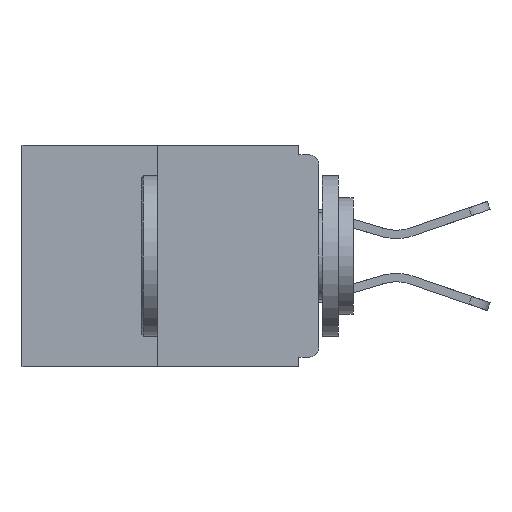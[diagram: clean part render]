
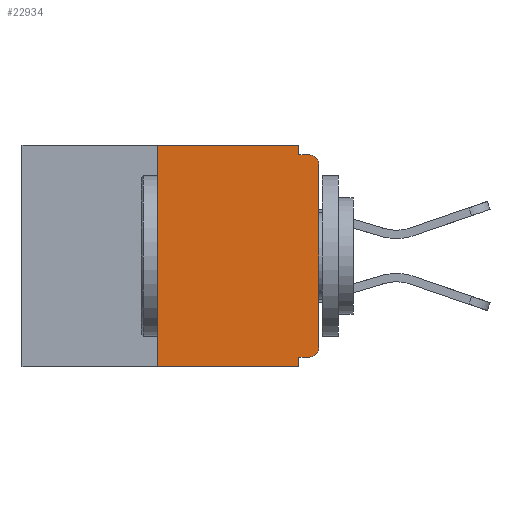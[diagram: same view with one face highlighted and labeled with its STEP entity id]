
A CAD part, left-side view. The second image highlights one B-rep face of the part: STEP entity #22934.
In plain terms, the highlighted planar face has unit normal (-1, 0, 0).
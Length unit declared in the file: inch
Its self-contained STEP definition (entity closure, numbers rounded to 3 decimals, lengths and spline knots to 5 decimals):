
#298 = ORIENTED_EDGE ( 'NONE', *, *, #27920, .F. ) ;
#643 = AXIS2_PLACEMENT_3D ( 'NONE', #21522, #7256, #24028 ) ;
#1594 = EDGE_CURVE ( 'NONE', #24351, #18713, #19865, .T. ) ;
#2471 = DIRECTION ( 'NONE',  ( 0., 0., 1. ) ) ;
#2542 = CARTESIAN_POINT ( 'NONE',  ( 0., 0., -0.015 ) ) ;
#2867 = CARTESIAN_POINT ( 'NONE',  ( 0., 0.46, -0.343 ) ) ;
#2940 = CARTESIAN_POINT ( 'NONE',  ( 0., 0.25, 0. ) ) ;
#3833 = VECTOR ( 'NONE', #12038, 39.37008 ) ;
#4502 = VERTEX_POINT ( 'NONE', #25814 ) ;
#4508 = DIRECTION ( 'NONE',  ( 0., 0., -1. ) ) ;
#5041 = LINE ( 'NONE', #2867, #21056 ) ;
#5176 = CARTESIAN_POINT ( 'NONE',  ( 0., 0., -0.328 ) ) ;
#5350 = LINE ( 'NONE', #2542, #3833 ) ;
#5552 = DIRECTION ( 'NONE',  ( 0., -1., 0. ) ) ;
#6161 = LINE ( 'NONE', #13397, #23680 ) ;
#6518 = EDGE_LOOP ( 'NONE', ( #11911, #21183, #27392, #6928, #298, #19689, #8273, #9486, #28168, #14621 ) ) ;
#6821 = VERTEX_POINT ( 'NONE', #10966 ) ;
#6928 = ORIENTED_EDGE ( 'NONE', *, *, #21513, .F. ) ;
#6950 = DIRECTION ( 'NONE',  ( -1., 0., 0. ) ) ;
#7131 = CARTESIAN_POINT ( 'NONE',  ( 0., 0., 0. ) ) ;
#7256 = DIRECTION ( 'NONE',  ( -1., 0., 0. ) ) ;
#7584 = VECTOR ( 'NONE', #14954, 39.37008 ) ;
#8237 = VERTEX_POINT ( 'NONE', #13868 ) ;
#8273 = ORIENTED_EDGE ( 'NONE', *, *, #19699, .T. ) ;
#8434 = CARTESIAN_POINT ( 'NONE',  ( 0., 0.015, -0.015 ) ) ;
#8556 = CARTESIAN_POINT ( 'NONE',  ( 0., 0.031, 0. ) ) ;
#8578 = CARTESIAN_POINT ( 'NONE',  ( 0., 0.46, 0. ) ) ;
#8872 = VERTEX_POINT ( 'NONE', #19354 ) ;
#9145 = CARTESIAN_POINT ( 'NONE',  ( 0., 0., -0.03 ) ) ;
#9486 = ORIENTED_EDGE ( 'NONE', *, *, #30631, .T. ) ;
#9489 = LINE ( 'NONE', #7131, #19171 ) ;
#10614 = VERTEX_POINT ( 'NONE', #28430 ) ;
#10966 = CARTESIAN_POINT ( 'NONE',  ( 0., 0., -0.313 ) ) ;
#11784 = EDGE_CURVE ( 'NONE', #19048, #8872, #14375, .T. ) ;
#11911 = ORIENTED_EDGE ( 'NONE', *, *, #26491, .F. ) ;
#11927 = CIRCLE ( 'NONE', #643, 0.015 ) ;
#12038 = DIRECTION ( 'NONE',  ( 0., -1., 0. ) ) ;
#12622 = DIRECTION ( 'NONE',  ( 0., 1., 0. ) ) ;
#13140 = CARTESIAN_POINT ( 'NONE',  ( 0., 0.25, 0. ) ) ;
#13221 = AXIS2_PLACEMENT_3D ( 'NONE', #21212, #6950, #23631 ) ;
#13397 = CARTESIAN_POINT ( 'NONE',  ( 0., 0.031, -0.343 ) ) ;
#13868 = CARTESIAN_POINT ( 'NONE',  ( 0., 0.031, -0.343 ) ) ;
#14261 = VERTEX_POINT ( 'NONE', #9145 ) ;
#14375 = LINE ( 'NONE', #15808, #20764 ) ;
#14544 = LINE ( 'NONE', #5176, #19390 ) ;
#14621 = ORIENTED_EDGE ( 'NONE', *, *, #11784, .F. ) ;
#14954 = DIRECTION ( 'NONE',  ( 0., 0., 1. ) ) ;
#15428 = DIRECTION ( 'NONE',  ( 0., 0., -1. ) ) ;
#15533 = DIRECTION ( 'NONE',  ( 1., 0., 0. ) ) ;
#15808 = CARTESIAN_POINT ( 'NONE',  ( 0., 0.031, 0. ) ) ;
#16171 = CARTESIAN_POINT ( 'NONE',  ( 0., 0.46, 0. ) ) ;
#17566 = CARTESIAN_POINT ( 'NONE',  ( 0., 0.25, -0.343 ) ) ;
#18573 = DIRECTION ( 'NONE',  ( 0., -1., 0. ) ) ;
#18713 = VERTEX_POINT ( 'NONE', #13140 ) ;
#18975 = LINE ( 'NONE', #16171, #23866 ) ;
#19048 = VERTEX_POINT ( 'NONE', #8556 ) ;
#19171 = VECTOR ( 'NONE', #2471, 39.37008 ) ;
#19354 = CARTESIAN_POINT ( 'NONE',  ( 0., 0.031, -0.015 ) ) ;
#19390 = VECTOR ( 'NONE', #12622, 39.37008 ) ;
#19689 = ORIENTED_EDGE ( 'NONE', *, *, #27826, .T. ) ;
#19699 = EDGE_CURVE ( 'NONE', #6821, #14261, #9489, .T. ) ;
#19865 = LINE ( 'NONE', #2940, #7584 ) ;
#20715 = DIRECTION ( 'NONE',  ( 0., 0., -1. ) ) ;
#20764 = VECTOR ( 'NONE', #4508, 39.37008 ) ;
#21056 = VECTOR ( 'NONE', #5552, 39.37008 ) ;
#21183 = ORIENTED_EDGE ( 'NONE', *, *, #1594, .F. ) ;
#21212 = CARTESIAN_POINT ( 'NONE',  ( 0., 0.015, -0.03 ) ) ;
#21298 = EDGE_CURVE ( 'NONE', #24351, #8237, #5041, .T. ) ;
#21513 = EDGE_CURVE ( 'NONE', #4502, #8237, #6161, .T. ) ;
#21522 = CARTESIAN_POINT ( 'NONE',  ( 0., 0.015, -0.313 ) ) ;
#21969 = CIRCLE ( 'NONE', #13221, 0.015 ) ;
#22934 = ADVANCED_FACE ( 'NONE', ( #26925 ), #30033, .F. ) ;
#23631 = DIRECTION ( 'NONE',  ( 0., 0., -1. ) ) ;
#23680 = VECTOR ( 'NONE', #20715, 39.37008 ) ;
#23866 = VECTOR ( 'NONE', #18573, 39.37008 ) ;
#24028 = DIRECTION ( 'NONE',  ( 0., 0., -1. ) ) ;
#24351 = VERTEX_POINT ( 'NONE', #17566 ) ;
#25814 = CARTESIAN_POINT ( 'NONE',  ( 0., 0.031, -0.328 ) ) ;
#26491 = EDGE_CURVE ( 'NONE', #18713, #19048, #18975, .T. ) ;
#26925 = FACE_OUTER_BOUND ( 'NONE', #6518, .T. ) ;
#26932 = EDGE_CURVE ( 'NONE', #8872, #29850, #5350, .T. ) ;
#27392 = ORIENTED_EDGE ( 'NONE', *, *, #21298, .T. ) ;
#27826 = EDGE_CURVE ( 'NONE', #10614, #6821, #11927, .T. ) ;
#27920 = EDGE_CURVE ( 'NONE', #10614, #4502, #14544, .T. ) ;
#28168 = ORIENTED_EDGE ( 'NONE', *, *, #26932, .F. ) ;
#28430 = CARTESIAN_POINT ( 'NONE',  ( 0., 0.015, -0.328 ) ) ;
#29850 = VERTEX_POINT ( 'NONE', #8434 ) ;
#30033 = PLANE ( 'NONE',  #30272 ) ;
#30272 = AXIS2_PLACEMENT_3D ( 'NONE', #8578, #15533, #15428 ) ;
#30631 = EDGE_CURVE ( 'NONE', #14261, #29850, #21969, .T. ) ;
